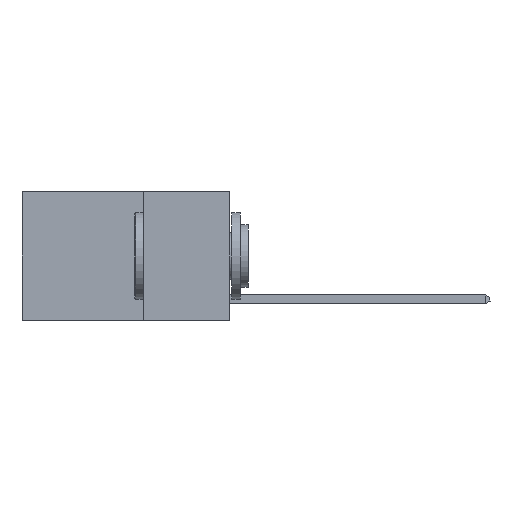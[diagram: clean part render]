
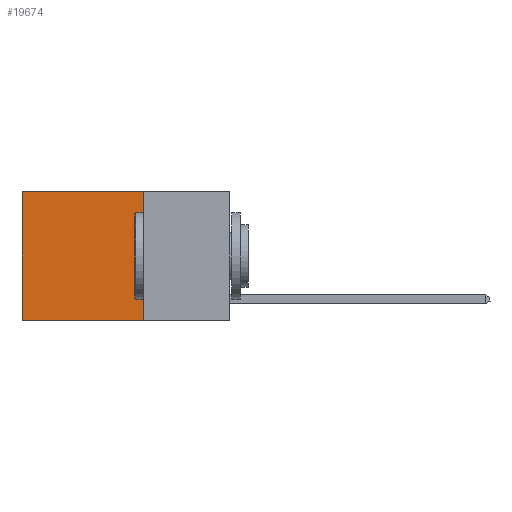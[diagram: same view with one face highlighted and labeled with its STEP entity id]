
A CAD part, left-side view. The second image highlights one B-rep face of the part: STEP entity #19674.
In plain terms, the highlighted planar face has unit normal (-1, 0, 0).
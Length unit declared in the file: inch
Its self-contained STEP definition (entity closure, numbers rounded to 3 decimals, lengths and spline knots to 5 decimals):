
#349 = DIRECTION ( 'NONE',  ( 0., 0., -1. ) ) ;
#2430 = EDGE_CURVE ( 'NONE', #8540, #25491, #26305, .T. ) ;
#4511 = DIRECTION ( 'NONE',  ( 0., 1., 0. ) ) ;
#5567 = VERTEX_POINT ( 'NONE', #27878 ) ;
#7047 = CARTESIAN_POINT ( 'NONE',  ( 0.2625, 0.25, 0. ) ) ;
#7288 = EDGE_CURVE ( 'NONE', #25491, #5567, #16044, .T. ) ;
#8305 = ORIENTED_EDGE ( 'NONE', *, *, #14224, .F. ) ;
#8540 = VERTEX_POINT ( 'NONE', #22910 ) ;
#8883 = LINE ( 'NONE', #26529, #19311 ) ;
#9144 = EDGE_LOOP ( 'NONE', ( #20259, #13654, #8305, #17464 ) ) ;
#9897 = VECTOR ( 'NONE', #24728, 39.37008 ) ;
#10370 = CARTESIAN_POINT ( 'NONE',  ( 0.2625, 0.6, 0. ) ) ;
#11930 = EDGE_CURVE ( 'NONE', #25123, #5567, #23529, .T. ) ;
#12656 = AXIS2_PLACEMENT_3D ( 'NONE', #19295, #25986, #27979 ) ;
#12694 = CARTESIAN_POINT ( 'NONE',  ( 0.2625, 0.25, -0.37 ) ) ;
#12956 = CARTESIAN_POINT ( 'NONE',  ( 0.2625, 0.25, -0.37 ) ) ;
#13654 = ORIENTED_EDGE ( 'NONE', *, *, #11930, .F. ) ;
#14224 = EDGE_CURVE ( 'NONE', #8540, #25123, #8883, .T. ) ;
#14321 = CARTESIAN_POINT ( 'NONE',  ( 0.2625, 0.6, 0. ) ) ;
#16044 = LINE ( 'NONE', #14321, #9897 ) ;
#17443 = FACE_OUTER_BOUND ( 'NONE', #9144, .T. ) ;
#17464 = ORIENTED_EDGE ( 'NONE', *, *, #2430, .T. ) ;
#19295 = CARTESIAN_POINT ( 'NONE',  ( 0.2625, 0.25, 0. ) ) ;
#19311 = VECTOR ( 'NONE', #349, 39.37008 ) ;
#19674 = ADVANCED_FACE ( 'NONE', ( #17443 ), #22009, .F. ) ;
#19907 = VECTOR ( 'NONE', #4511, 39.37008 ) ;
#20259 = ORIENTED_EDGE ( 'NONE', *, *, #7288, .T. ) ;
#21115 = DIRECTION ( 'NONE',  ( 0., 1., 0. ) ) ;
#22009 = PLANE ( 'NONE',  #12656 ) ;
#22910 = CARTESIAN_POINT ( 'NONE',  ( 0.2625, 0.25, 0. ) ) ;
#23529 = LINE ( 'NONE', #12694, #25706 ) ;
#24728 = DIRECTION ( 'NONE',  ( 0., 0., -1. ) ) ;
#25123 = VERTEX_POINT ( 'NONE', #12956 ) ;
#25491 = VERTEX_POINT ( 'NONE', #10370 ) ;
#25706 = VECTOR ( 'NONE', #21115, 39.37008 ) ;
#25986 = DIRECTION ( 'NONE',  ( 1., 0., 0. ) ) ;
#26305 = LINE ( 'NONE', #7047, #19907 ) ;
#26529 = CARTESIAN_POINT ( 'NONE',  ( 0.2625, 0.25, 0. ) ) ;
#27878 = CARTESIAN_POINT ( 'NONE',  ( 0.2625, 0.6, -0.37 ) ) ;
#27979 = DIRECTION ( 'NONE',  ( 0., 0., -1. ) ) ;
